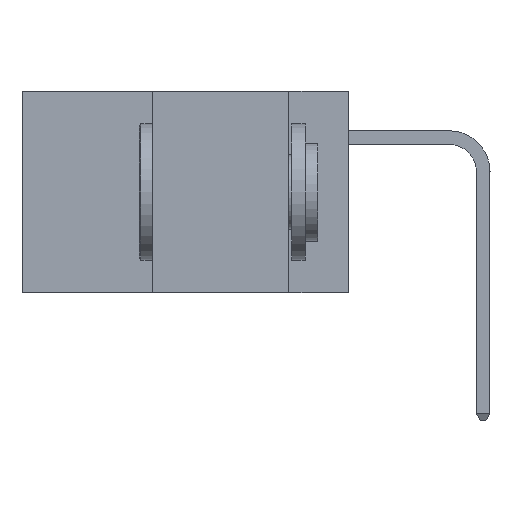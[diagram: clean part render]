
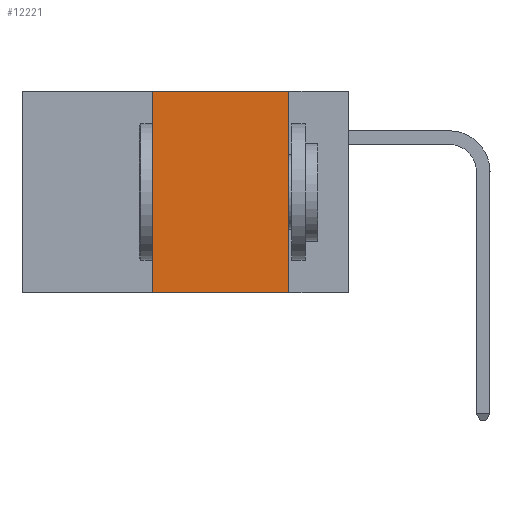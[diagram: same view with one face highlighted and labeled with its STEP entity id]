
A CAD part, left-side view. The second image highlights one B-rep face of the part: STEP entity #12221.
In plain terms, the highlighted planar face has unit normal (-1, 0, 0).
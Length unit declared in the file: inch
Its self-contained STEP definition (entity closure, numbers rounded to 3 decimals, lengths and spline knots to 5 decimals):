
#404 = CARTESIAN_POINT ( 'NONE',  ( 0., 0.11, 0. ) ) ;
#1130 = VERTEX_POINT ( 'NONE', #8710 ) ;
#1423 = VECTOR ( 'NONE', #15323, 39.37008 ) ;
#1535 = DIRECTION ( 'NONE',  ( 1., 0., 0. ) ) ;
#2721 = DIRECTION ( 'NONE',  ( 0., 0., 1. ) ) ;
#3103 = EDGE_CURVE ( 'NONE', #10743, #4546, #6093, .T. ) ;
#3416 = DIRECTION ( 'NONE',  ( 0., 0., -1. ) ) ;
#4155 = AXIS2_PLACEMENT_3D ( 'NONE', #21166, #1535, #13166 ) ;
#4317 = CARTESIAN_POINT ( 'NONE',  ( 0., 0.36, 0. ) ) ;
#4546 = VERTEX_POINT ( 'NONE', #404 ) ;
#4769 = ORIENTED_EDGE ( 'NONE', *, *, #3103, .F. ) ;
#4797 = LINE ( 'NONE', #4317, #13092 ) ;
#5277 = ORIENTED_EDGE ( 'NONE', *, *, #12688, .F. ) ;
#5611 = VECTOR ( 'NONE', #3416, 39.37008 ) ;
#5867 = LINE ( 'NONE', #12056, #1423 ) ;
#5981 = EDGE_LOOP ( 'NONE', ( #17359, #4769, #5277, #10279 ) ) ;
#6093 = LINE ( 'NONE', #10706, #14894 ) ;
#7403 = VERTEX_POINT ( 'NONE', #10398 ) ;
#8710 = CARTESIAN_POINT ( 'NONE',  ( 0., 0.11, -0.37 ) ) ;
#9057 = LINE ( 'NONE', #13336, #5611 ) ;
#10279 = ORIENTED_EDGE ( 'NONE', *, *, #11767, .T. ) ;
#10398 = CARTESIAN_POINT ( 'NONE',  ( 0., 0.36, -0.37 ) ) ;
#10706 = CARTESIAN_POINT ( 'NONE',  ( 0., 0.6, 0. ) ) ;
#10743 = VERTEX_POINT ( 'NONE', #20662 ) ;
#10847 = DIRECTION ( 'NONE',  ( 0., -1., 0. ) ) ;
#11610 = EDGE_CURVE ( 'NONE', #4546, #1130, #9057, .T. ) ;
#11767 = EDGE_CURVE ( 'NONE', #7403, #1130, #5867, .T. ) ;
#12056 = CARTESIAN_POINT ( 'NONE',  ( 0., 0.6, -0.37 ) ) ;
#12221 = ADVANCED_FACE ( 'NONE', ( #17900 ), #19568, .F. ) ;
#12688 = EDGE_CURVE ( 'NONE', #7403, #10743, #4797, .T. ) ;
#13092 = VECTOR ( 'NONE', #2721, 39.37008 ) ;
#13166 = DIRECTION ( 'NONE',  ( 0., 0., -1. ) ) ;
#13336 = CARTESIAN_POINT ( 'NONE',  ( 0., 0.11, 0. ) ) ;
#14894 = VECTOR ( 'NONE', #10847, 39.37008 ) ;
#15323 = DIRECTION ( 'NONE',  ( 0., -1., 0. ) ) ;
#17359 = ORIENTED_EDGE ( 'NONE', *, *, #11610, .F. ) ;
#17900 = FACE_OUTER_BOUND ( 'NONE', #5981, .T. ) ;
#19568 = PLANE ( 'NONE',  #4155 ) ;
#20662 = CARTESIAN_POINT ( 'NONE',  ( 0., 0.36, 0. ) ) ;
#21166 = CARTESIAN_POINT ( 'NONE',  ( 0., 0.6, 0. ) ) ;
